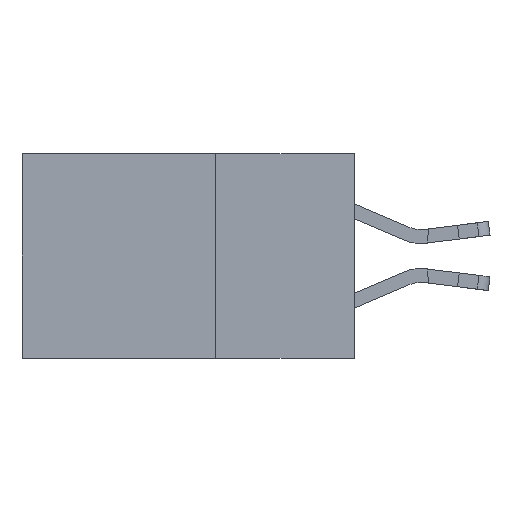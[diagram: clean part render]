
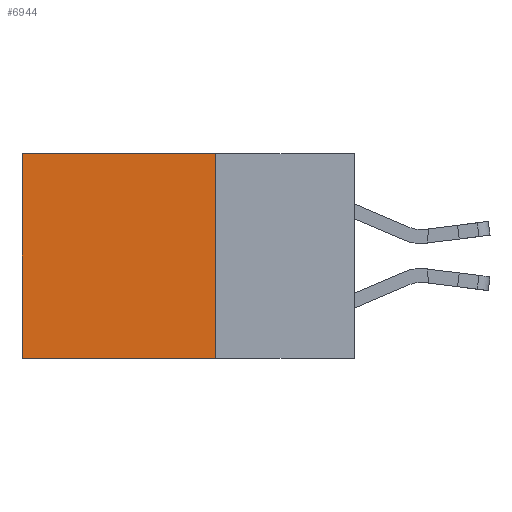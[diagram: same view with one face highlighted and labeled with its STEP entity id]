
A CAD part, left-side view. The second image highlights one B-rep face of the part: STEP entity #6944.
In plain terms, the highlighted planar face has unit normal (-1, 0, 0).
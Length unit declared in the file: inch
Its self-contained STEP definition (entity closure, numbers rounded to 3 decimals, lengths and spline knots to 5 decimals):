
#1 = DIRECTION ( 'NONE',  ( 0., 0., -1. ) ) ;
#231 = VECTOR ( 'NONE', #672, 39.37008 ) ;
#473 = ORIENTED_EDGE ( 'NONE', *, *, #9532, .T. ) ;
#672 = DIRECTION ( 'NONE',  ( 0., 1., 0. ) ) ;
#968 = ORIENTED_EDGE ( 'NONE', *, *, #4883, .T. ) ;
#1435 = ORIENTED_EDGE ( 'NONE', *, *, #2820, .F. ) ;
#1562 = CARTESIAN_POINT ( 'NONE',  ( 0.298, 0.25, 0. ) ) ;
#2328 = DIRECTION ( 'NONE',  ( 1., 0., 0. ) ) ;
#2820 = EDGE_CURVE ( 'NONE', #5615, #3424, #12790, .T. ) ;
#3077 = CARTESIAN_POINT ( 'NONE',  ( 0.298, 0.25, 0. ) ) ;
#3327 = LINE ( 'NONE', #6473, #231 ) ;
#3424 = VERTEX_POINT ( 'NONE', #9511 ) ;
#3905 = FACE_OUTER_BOUND ( 'NONE', #5222, .T. ) ;
#4011 = DIRECTION ( 'NONE',  ( 0., 0., -1. ) ) ;
#4883 = EDGE_CURVE ( 'NONE', #5615, #8409, #3327, .T. ) ;
#4913 = DIRECTION ( 'NONE',  ( 0., 1., 0. ) ) ;
#5222 = EDGE_LOOP ( 'NONE', ( #473, #14699, #1435, #968 ) ) ;
#5275 = LINE ( 'NONE', #7185, #10954 ) ;
#5615 = VERTEX_POINT ( 'NONE', #3077 ) ;
#5771 = PLANE ( 'NONE',  #13992 ) ;
#6473 = CARTESIAN_POINT ( 'NONE',  ( 0.298, 0.25, 0. ) ) ;
#6944 = ADVANCED_FACE ( 'NONE', ( #3905 ), #5771, .F. ) ;
#7185 = CARTESIAN_POINT ( 'NONE',  ( 0.298, 0.25, -0.37 ) ) ;
#7986 = VECTOR ( 'NONE', #1, 39.37008 ) ;
#8134 = CARTESIAN_POINT ( 'NONE',  ( 0.298, 0.6, 0. ) ) ;
#8409 = VERTEX_POINT ( 'NONE', #11601 ) ;
#9186 = CARTESIAN_POINT ( 'NONE',  ( 0.298, 0.25, 0. ) ) ;
#9511 = CARTESIAN_POINT ( 'NONE',  ( 0.298, 0.25, -0.37 ) ) ;
#9532 = EDGE_CURVE ( 'NONE', #8409, #13084, #13210, .T. ) ;
#9810 = CARTESIAN_POINT ( 'NONE',  ( 0.298, 0.6, -0.37 ) ) ;
#9843 = VECTOR ( 'NONE', #4011, 39.37008 ) ;
#10333 = DIRECTION ( 'NONE',  ( 0., 0., -1. ) ) ;
#10356 = EDGE_CURVE ( 'NONE', #3424, #13084, #5275, .T. ) ;
#10954 = VECTOR ( 'NONE', #4913, 39.37008 ) ;
#11601 = CARTESIAN_POINT ( 'NONE',  ( 0.298, 0.6, 0. ) ) ;
#12790 = LINE ( 'NONE', #1562, #9843 ) ;
#13084 = VERTEX_POINT ( 'NONE', #9810 ) ;
#13210 = LINE ( 'NONE', #8134, #7986 ) ;
#13992 = AXIS2_PLACEMENT_3D ( 'NONE', #9186, #2328, #10333 ) ;
#14699 = ORIENTED_EDGE ( 'NONE', *, *, #10356, .F. ) ;
